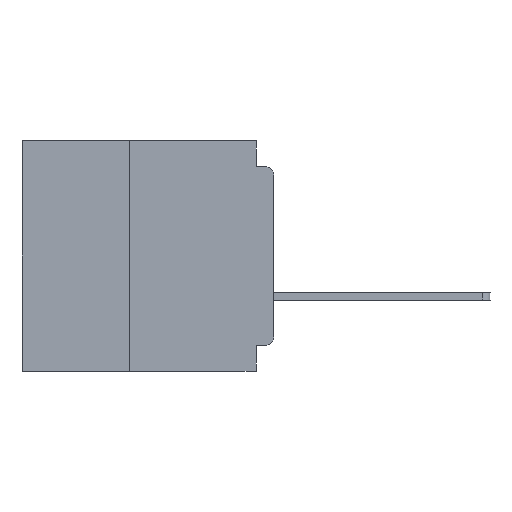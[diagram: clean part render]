
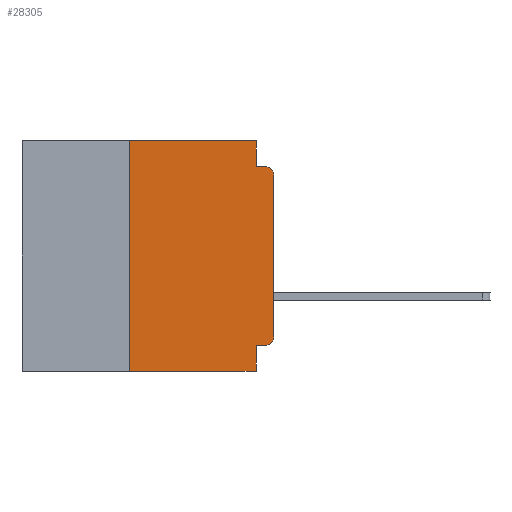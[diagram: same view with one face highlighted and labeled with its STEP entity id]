
A CAD part, left-side view. The second image highlights one B-rep face of the part: STEP entity #28305.
In plain terms, the highlighted planar face has unit normal (-1, 0, 0).
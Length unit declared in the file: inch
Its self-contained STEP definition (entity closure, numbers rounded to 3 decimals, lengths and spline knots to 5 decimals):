
#2404 = AXIS2_PLACEMENT_3D ( 'NONE', #26623, #11144, #47447 ) ;
#2754 = LINE ( 'NONE', #59560, #28831 ) ;
#3237 = VECTOR ( 'NONE', #14531, 39.37008 ) ;
#4401 = DIRECTION ( 'NONE',  ( 0., 0., -1. ) ) ;
#5891 = LINE ( 'NONE', #27167, #44025 ) ;
#5971 = EDGE_CURVE ( 'NONE', #15326, #52783, #48927, .T. ) ;
#7778 = CARTESIAN_POINT ( 'NONE',  ( 0., 0.015, -0.045 ) ) ;
#8306 = EDGE_LOOP ( 'NONE', ( #41680, #44490, #28470, #61708, #60015, #63214, #62508, #18083, #33840, #10613 ) ) ;
#8949 = CARTESIAN_POINT ( 'NONE',  ( 0., 0.031, -0.045 ) ) ;
#9079 = VECTOR ( 'NONE', #55408, 39.37008 ) ;
#9429 = EDGE_CURVE ( 'NONE', #9773, #61063, #56790, .T. ) ;
#9773 = VERTEX_POINT ( 'NONE', #22697 ) ;
#9983 = LINE ( 'NONE', #58917, #51389 ) ;
#10613 = ORIENTED_EDGE ( 'NONE', *, *, #5971, .T. ) ;
#11144 = DIRECTION ( 'NONE',  ( 1., 0., 0. ) ) ;
#11293 = CARTESIAN_POINT ( 'NONE',  ( 0., 0.031, 0. ) ) ;
#13314 = CARTESIAN_POINT ( 'NONE',  ( 0., 0.031, -0.4 ) ) ;
#14531 = DIRECTION ( 'NONE',  ( 0., -1., 0. ) ) ;
#14708 = EDGE_CURVE ( 'NONE', #63703, #9773, #22923, .T. ) ;
#15326 = VERTEX_POINT ( 'NONE', #55101 ) ;
#18083 = ORIENTED_EDGE ( 'NONE', *, *, #46948, .F. ) ;
#18938 = EDGE_CURVE ( 'NONE', #15326, #29334, #2754, .T. ) ;
#19404 = CARTESIAN_POINT ( 'NONE',  ( 0., 0., 0. ) ) ;
#22697 = CARTESIAN_POINT ( 'NONE',  ( 0., 0.25, 0. ) ) ;
#22923 = LINE ( 'NONE', #34405, #9079 ) ;
#23629 = EDGE_CURVE ( 'NONE', #64609, #40590, #9983, .T. ) ;
#24257 = CARTESIAN_POINT ( 'NONE',  ( 0., 0.015, -0.34 ) ) ;
#24642 = EDGE_CURVE ( 'NONE', #63703, #66790, #5891, .T. ) ;
#24657 = CARTESIAN_POINT ( 'NONE',  ( 0., 0.031, -0.355 ) ) ;
#26623 = CARTESIAN_POINT ( 'NONE',  ( 0., 0.437, 0. ) ) ;
#27167 = CARTESIAN_POINT ( 'NONE',  ( 0., 0.437, -0.4 ) ) ;
#27963 = DIRECTION ( 'NONE',  ( 0., -1., 0. ) ) ;
#28305 = ADVANCED_FACE ( 'NONE', ( #55657 ), #42210, .F. ) ;
#28470 = ORIENTED_EDGE ( 'NONE', *, *, #23629, .F. ) ;
#28831 = VECTOR ( 'NONE', #49190, 39.37008 ) ;
#29334 = VERTEX_POINT ( 'NONE', #24657 ) ;
#29475 = DIRECTION ( 'NONE',  ( 0., 0., -1. ) ) ;
#30127 = AXIS2_PLACEMENT_3D ( 'NONE', #66447, #35509, #4401 ) ;
#32355 = CARTESIAN_POINT ( 'NONE',  ( 0., 0., -0.06 ) ) ;
#32362 = DIRECTION ( 'NONE',  ( 0., -1., 0. ) ) ;
#32424 = AXIS2_PLACEMENT_3D ( 'NONE', #24257, #60423, #29475 ) ;
#32684 = CARTESIAN_POINT ( 'NONE',  ( 0., 0.25, -0.4 ) ) ;
#33840 = ORIENTED_EDGE ( 'NONE', *, *, #18938, .F. ) ;
#34405 = CARTESIAN_POINT ( 'NONE',  ( 0., 0.25, -0.4 ) ) ;
#34693 = EDGE_CURVE ( 'NONE', #44283, #40590, #66733, .T. ) ;
#35509 = DIRECTION ( 'NONE',  ( -1., 0., 0. ) ) ;
#35733 = CARTESIAN_POINT ( 'NONE',  ( 0., 0.031, 0. ) ) ;
#40590 = VERTEX_POINT ( 'NONE', #7778 ) ;
#41680 = ORIENTED_EDGE ( 'NONE', *, *, #64616, .T. ) ;
#42070 = CARTESIAN_POINT ( 'NONE',  ( 0., 0.031, -0.4 ) ) ;
#42210 = PLANE ( 'NONE',  #2404 ) ;
#43155 = VECTOR ( 'NONE', #52770, 39.37008 ) ;
#44025 = VECTOR ( 'NONE', #32362, 39.37008 ) ;
#44283 = VERTEX_POINT ( 'NONE', #32355 ) ;
#44490 = ORIENTED_EDGE ( 'NONE', *, *, #34693, .T. ) ;
#44795 = LINE ( 'NONE', #11293, #43155 ) ;
#45617 = CARTESIAN_POINT ( 'NONE',  ( 0., 0.437, 0. ) ) ;
#46948 = EDGE_CURVE ( 'NONE', #29334, #66790, #47492, .T. ) ;
#47447 = DIRECTION ( 'NONE',  ( 0., 0., -1. ) ) ;
#47492 = LINE ( 'NONE', #42070, #59586 ) ;
#48927 = CIRCLE ( 'NONE', #32424, 0.015 ) ;
#49143 = VECTOR ( 'NONE', #66000, 39.37008 ) ;
#49190 = DIRECTION ( 'NONE',  ( 0., 1., 0. ) ) ;
#51389 = VECTOR ( 'NONE', #27963, 39.37008 ) ;
#52770 = DIRECTION ( 'NONE',  ( 0., 0., -1. ) ) ;
#52783 = VERTEX_POINT ( 'NONE', #59049 ) ;
#55101 = CARTESIAN_POINT ( 'NONE',  ( 0., 0.015, -0.355 ) ) ;
#55408 = DIRECTION ( 'NONE',  ( 0., 0., 1. ) ) ;
#55657 = FACE_OUTER_BOUND ( 'NONE', #8306, .T. ) ;
#56790 = LINE ( 'NONE', #45617, #3237 ) ;
#58917 = CARTESIAN_POINT ( 'NONE',  ( 0., 0., -0.045 ) ) ;
#59049 = CARTESIAN_POINT ( 'NONE',  ( 0., 0., -0.34 ) ) ;
#59560 = CARTESIAN_POINT ( 'NONE',  ( 0., 0., -0.355 ) ) ;
#59586 = VECTOR ( 'NONE', #62648, 39.37008 ) ;
#60015 = ORIENTED_EDGE ( 'NONE', *, *, #9429, .F. ) ;
#60423 = DIRECTION ( 'NONE',  ( -1., 0., 0. ) ) ;
#61063 = VERTEX_POINT ( 'NONE', #35733 ) ;
#61708 = ORIENTED_EDGE ( 'NONE', *, *, #66563, .F. ) ;
#62508 = ORIENTED_EDGE ( 'NONE', *, *, #24642, .T. ) ;
#62648 = DIRECTION ( 'NONE',  ( 0., 0., -1. ) ) ;
#63214 = ORIENTED_EDGE ( 'NONE', *, *, #14708, .F. ) ;
#63703 = VERTEX_POINT ( 'NONE', #32684 ) ;
#64609 = VERTEX_POINT ( 'NONE', #8949 ) ;
#64616 = EDGE_CURVE ( 'NONE', #52783, #44283, #66102, .T. ) ;
#66000 = DIRECTION ( 'NONE',  ( 0., 0., 1. ) ) ;
#66102 = LINE ( 'NONE', #19404, #49143 ) ;
#66447 = CARTESIAN_POINT ( 'NONE',  ( 0., 0.015, -0.06 ) ) ;
#66563 = EDGE_CURVE ( 'NONE', #61063, #64609, #44795, .T. ) ;
#66733 = CIRCLE ( 'NONE', #30127, 0.015 ) ;
#66790 = VERTEX_POINT ( 'NONE', #13314 ) ;
